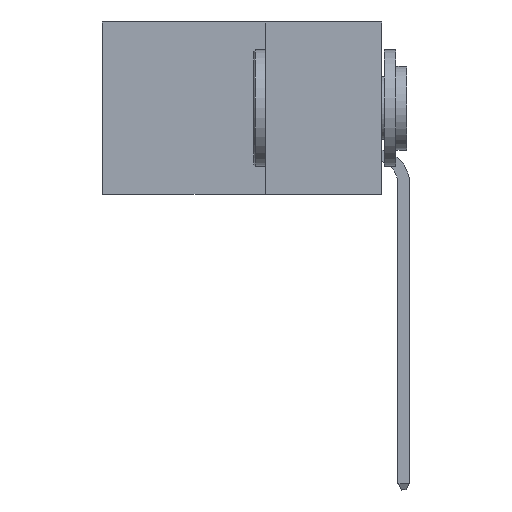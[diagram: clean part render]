
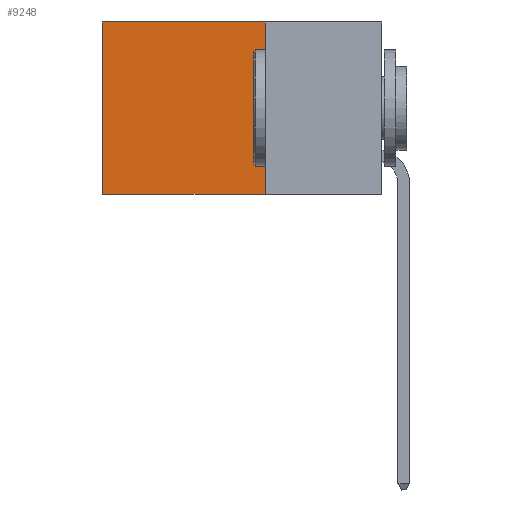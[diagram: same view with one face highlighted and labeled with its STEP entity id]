
A CAD part, left-side view. The second image highlights one B-rep face of the part: STEP entity #9248.
In plain terms, the highlighted planar face has unit normal (-1, 0, 0).
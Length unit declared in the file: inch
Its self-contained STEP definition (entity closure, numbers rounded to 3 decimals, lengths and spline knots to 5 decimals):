
#1610 = DIRECTION ( 'NONE',  ( 0., 0., -1. ) ) ;
#2056 = ORIENTED_EDGE ( 'NONE', *, *, #16629, .F. ) ;
#2309 = DIRECTION ( 'NONE',  ( 0., 1., 0. ) ) ;
#2714 = LINE ( 'NONE', #22691, #14477 ) ;
#2950 = EDGE_LOOP ( 'NONE', ( #11428, #26216, #2056, #9951 ) ) ;
#3846 = VECTOR ( 'NONE', #26396, 39.37008 ) ;
#4746 = CARTESIAN_POINT ( 'NONE',  ( 0.2875, 0.25, 0. ) ) ;
#4813 = VERTEX_POINT ( 'NONE', #23137 ) ;
#4924 = FACE_OUTER_BOUND ( 'NONE', #2950, .T. ) ;
#4989 = CARTESIAN_POINT ( 'NONE',  ( 0.2875, 0.6, 0. ) ) ;
#7832 = VERTEX_POINT ( 'NONE', #22034 ) ;
#9248 = ADVANCED_FACE ( 'NONE', ( #4924 ), #9971, .F. ) ;
#9440 = DIRECTION ( 'NONE',  ( 0., 0., -1. ) ) ;
#9884 = CARTESIAN_POINT ( 'NONE',  ( 0.2875, 0.25, 0. ) ) ;
#9951 = ORIENTED_EDGE ( 'NONE', *, *, #17820, .T. ) ;
#9971 = PLANE ( 'NONE',  #14136 ) ;
#11428 = ORIENTED_EDGE ( 'NONE', *, *, #23726, .T. ) ;
#12002 = LINE ( 'NONE', #15419, #12661 ) ;
#12288 = DIRECTION ( 'NONE',  ( 1., 0., 0. ) ) ;
#12661 = VECTOR ( 'NONE', #9440, 39.37008 ) ;
#13474 = CARTESIAN_POINT ( 'NONE',  ( 0.2875, 0.25, -0.37 ) ) ;
#14136 = AXIS2_PLACEMENT_3D ( 'NONE', #9884, #12288, #1610 ) ;
#14477 = VECTOR ( 'NONE', #26843, 39.37008 ) ;
#15009 = VECTOR ( 'NONE', #2309, 39.37008 ) ;
#15419 = CARTESIAN_POINT ( 'NONE',  ( 0.2875, 0.25, 0. ) ) ;
#15591 = LINE ( 'NONE', #13474, #3846 ) ;
#16629 = EDGE_CURVE ( 'NONE', #4813, #7832, #12002, .T. ) ;
#17820 = EDGE_CURVE ( 'NONE', #4813, #24492, #23990, .T. ) ;
#19545 = CARTESIAN_POINT ( 'NONE',  ( 0.2875, 0.6, -0.37 ) ) ;
#20805 = VERTEX_POINT ( 'NONE', #19545 ) ;
#22034 = CARTESIAN_POINT ( 'NONE',  ( 0.2875, 0.25, -0.37 ) ) ;
#22068 = EDGE_CURVE ( 'NONE', #7832, #20805, #15591, .T. ) ;
#22691 = CARTESIAN_POINT ( 'NONE',  ( 0.2875, 0.6, 0. ) ) ;
#23137 = CARTESIAN_POINT ( 'NONE',  ( 0.2875, 0.25, 0. ) ) ;
#23726 = EDGE_CURVE ( 'NONE', #24492, #20805, #2714, .T. ) ;
#23990 = LINE ( 'NONE', #4746, #15009 ) ;
#24492 = VERTEX_POINT ( 'NONE', #4989 ) ;
#26216 = ORIENTED_EDGE ( 'NONE', *, *, #22068, .F. ) ;
#26396 = DIRECTION ( 'NONE',  ( 0., 1., 0. ) ) ;
#26843 = DIRECTION ( 'NONE',  ( 0., 0., -1. ) ) ;
